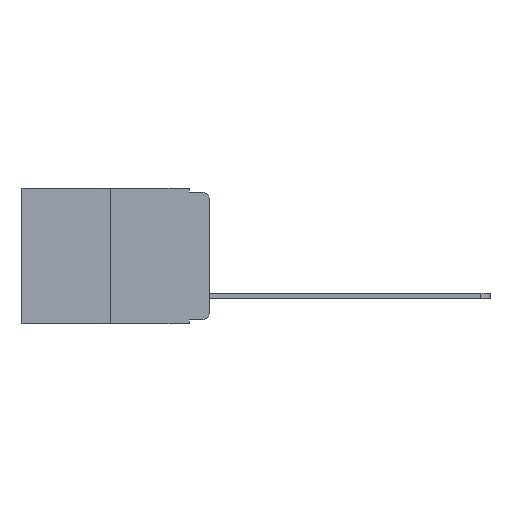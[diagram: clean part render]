
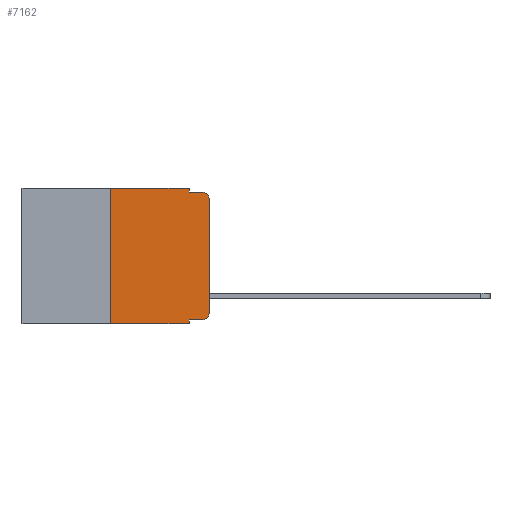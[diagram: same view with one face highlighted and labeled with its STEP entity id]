
A CAD part, left-side view. The second image highlights one B-rep face of the part: STEP entity #7162.
In plain terms, the highlighted planar face has unit normal (-1, 0, 0).
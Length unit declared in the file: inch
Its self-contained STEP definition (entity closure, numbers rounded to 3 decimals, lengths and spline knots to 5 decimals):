
#19 = EDGE_CURVE ( 'NONE', #10190, #10269, #2361, .T. ) ;
#257 = DIRECTION ( 'NONE',  ( -1., 0., 0. ) ) ;
#281 = VERTEX_POINT ( 'NONE', #7992 ) ;
#346 = CARTESIAN_POINT ( 'NONE',  ( 0., 0.051, 0. ) ) ;
#434 = VECTOR ( 'NONE', #2835, 39.37008 ) ;
#930 = CARTESIAN_POINT ( 'NONE',  ( 0., 0.02, -0.01 ) ) ;
#1138 = DIRECTION ( 'NONE',  ( 0., -1., 0. ) ) ;
#1669 = DIRECTION ( 'NONE',  ( 0., -1., 0. ) ) ;
#1837 = CARTESIAN_POINT ( 'NONE',  ( 0., 0.473, 0. ) ) ;
#2078 = VERTEX_POINT ( 'NONE', #12158 ) ;
#2218 = CARTESIAN_POINT ( 'NONE',  ( 0., 0.02, -0.03 ) ) ;
#2294 = CARTESIAN_POINT ( 'NONE',  ( 0., 0.473, -0.343 ) ) ;
#2296 = VECTOR ( 'NONE', #1138, 39.37008 ) ;
#2299 = EDGE_CURVE ( 'NONE', #10269, #7251, #5042, .T. ) ;
#2361 = LINE ( 'NONE', #346, #12583 ) ;
#2375 = VERTEX_POINT ( 'NONE', #5744 ) ;
#2410 = VECTOR ( 'NONE', #7650, 39.37008 ) ;
#2417 = VERTEX_POINT ( 'NONE', #6441 ) ;
#2548 = DIRECTION ( 'NONE',  ( 0., 0., -1. ) ) ;
#2632 = CIRCLE ( 'NONE', #8347, 0.02 ) ;
#2835 = DIRECTION ( 'NONE',  ( 0., 0., -1. ) ) ;
#2884 = PLANE ( 'NONE',  #9440 ) ;
#3189 = FACE_OUTER_BOUND ( 'NONE', #7065, .T. ) ;
#3408 = VECTOR ( 'NONE', #3560, 39.37008 ) ;
#3560 = DIRECTION ( 'NONE',  ( 0., 0., 1. ) ) ;
#3673 = EDGE_CURVE ( 'NONE', #2417, #7251, #2632, .T. ) ;
#3758 = CIRCLE ( 'NONE', #10179, 0.02 ) ;
#3819 = CARTESIAN_POINT ( 'NONE',  ( 0., 0.051, 0. ) ) ;
#4015 = EDGE_CURVE ( 'NONE', #2078, #5225, #12664, .T. ) ;
#4343 = EDGE_CURVE ( 'NONE', #5190, #2417, #6146, .T. ) ;
#4569 = DIRECTION ( 'NONE',  ( 0., -1., 0. ) ) ;
#4908 = DIRECTION ( 'NONE',  ( -1., 0., 0. ) ) ;
#4964 = DIRECTION ( 'NONE',  ( 0., 0., -1. ) ) ;
#5042 = LINE ( 'NONE', #10245, #2296 ) ;
#5153 = LINE ( 'NONE', #5574, #2410 ) ;
#5190 = VERTEX_POINT ( 'NONE', #12773 ) ;
#5225 = VERTEX_POINT ( 'NONE', #7205 ) ;
#5325 = ORIENTED_EDGE ( 'NONE', *, *, #4343, .T. ) ;
#5513 = ORIENTED_EDGE ( 'NONE', *, *, #3673, .T. ) ;
#5574 = CARTESIAN_POINT ( 'NONE',  ( 0., 0.051, -0.333 ) ) ;
#5744 = CARTESIAN_POINT ( 'NONE',  ( 0., 0.25, 0. ) ) ;
#5789 = ORIENTED_EDGE ( 'NONE', *, *, #2299, .F. ) ;
#6082 = LINE ( 'NONE', #3819, #434 ) ;
#6146 = LINE ( 'NONE', #8792, #3408 ) ;
#6259 = ORIENTED_EDGE ( 'NONE', *, *, #19, .F. ) ;
#6359 = VECTOR ( 'NONE', #4569, 39.37008 ) ;
#6410 = ORIENTED_EDGE ( 'NONE', *, *, #12530, .F. ) ;
#6441 = CARTESIAN_POINT ( 'NONE',  ( 0., 0., -0.03 ) ) ;
#6476 = ORIENTED_EDGE ( 'NONE', *, *, #11297, .F. ) ;
#6545 = VECTOR ( 'NONE', #9558, 39.37008 ) ;
#6574 = VERTEX_POINT ( 'NONE', #12658 ) ;
#6613 = CARTESIAN_POINT ( 'NONE',  ( 0., 0.02, -0.313 ) ) ;
#6687 = LINE ( 'NONE', #12442, #6359 ) ;
#7065 = EDGE_LOOP ( 'NONE', ( #5325, #5513, #5789, #6259, #6410, #6476, #7164, #10005, #10116, #10358 ) ) ;
#7162 = ADVANCED_FACE ( 'NONE', ( #3189 ), #2884, .F. ) ;
#7164 = ORIENTED_EDGE ( 'NONE', *, *, #4015, .T. ) ;
#7205 = CARTESIAN_POINT ( 'NONE',  ( 0., 0.051, -0.343 ) ) ;
#7251 = VERTEX_POINT ( 'NONE', #930 ) ;
#7268 = VECTOR ( 'NONE', #1669, 39.37008 ) ;
#7621 = DIRECTION ( 'NONE',  ( 0., 0., -1. ) ) ;
#7650 = DIRECTION ( 'NONE',  ( 0., -1., 0. ) ) ;
#7795 = LINE ( 'NONE', #8568, #6545 ) ;
#7992 = CARTESIAN_POINT ( 'NONE',  ( 0., 0.051, -0.333 ) ) ;
#8347 = AXIS2_PLACEMENT_3D ( 'NONE', #2218, #4908, #2548 ) ;
#8568 = CARTESIAN_POINT ( 'NONE',  ( 0., 0.25, 0. ) ) ;
#8792 = CARTESIAN_POINT ( 'NONE',  ( 0., 0., 0. ) ) ;
#9370 = EDGE_CURVE ( 'NONE', #6574, #5190, #3758, .T. ) ;
#9440 = AXIS2_PLACEMENT_3D ( 'NONE', #1837, #10936, #4964 ) ;
#9558 = DIRECTION ( 'NONE',  ( 0., 0., 1. ) ) ;
#9988 = EDGE_CURVE ( 'NONE', #281, #6574, #5153, .T. ) ;
#10005 = ORIENTED_EDGE ( 'NONE', *, *, #10672, .F. ) ;
#10114 = CARTESIAN_POINT ( 'NONE',  ( 0., 0.051, -0.01 ) ) ;
#10116 = ORIENTED_EDGE ( 'NONE', *, *, #9988, .T. ) ;
#10179 = AXIS2_PLACEMENT_3D ( 'NONE', #6613, #257, #7621 ) ;
#10190 = VERTEX_POINT ( 'NONE', #11883 ) ;
#10245 = CARTESIAN_POINT ( 'NONE',  ( 0., 0.051, -0.01 ) ) ;
#10269 = VERTEX_POINT ( 'NONE', #10114 ) ;
#10358 = ORIENTED_EDGE ( 'NONE', *, *, #9370, .T. ) ;
#10672 = EDGE_CURVE ( 'NONE', #281, #5225, #6082, .T. ) ;
#10936 = DIRECTION ( 'NONE',  ( 1., 0., 0. ) ) ;
#11297 = EDGE_CURVE ( 'NONE', #2078, #2375, #7795, .T. ) ;
#11883 = CARTESIAN_POINT ( 'NONE',  ( 0., 0.051, 0. ) ) ;
#12158 = CARTESIAN_POINT ( 'NONE',  ( 0., 0.25, -0.343 ) ) ;
#12169 = DIRECTION ( 'NONE',  ( 0., 0., -1. ) ) ;
#12442 = CARTESIAN_POINT ( 'NONE',  ( 0., 0.473, 0. ) ) ;
#12530 = EDGE_CURVE ( 'NONE', #2375, #10190, #6687, .T. ) ;
#12583 = VECTOR ( 'NONE', #12169, 39.37008 ) ;
#12658 = CARTESIAN_POINT ( 'NONE',  ( 0., 0.02, -0.333 ) ) ;
#12664 = LINE ( 'NONE', #2294, #7268 ) ;
#12773 = CARTESIAN_POINT ( 'NONE',  ( 0., 0., -0.313 ) ) ;
